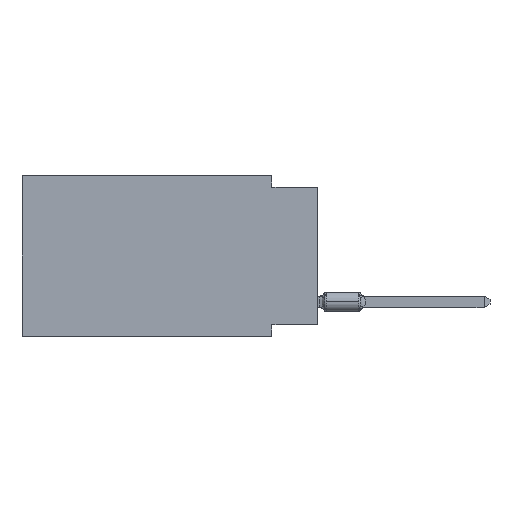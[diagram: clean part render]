
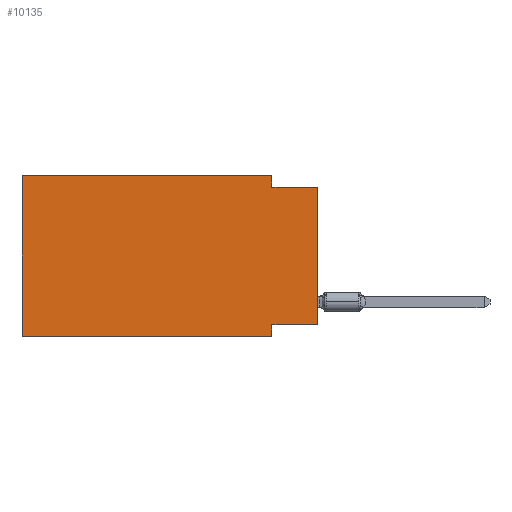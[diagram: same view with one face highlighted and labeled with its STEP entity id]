
A CAD part, left-side view. The second image highlights one B-rep face of the part: STEP entity #10135.
In plain terms, the highlighted planar face has unit normal (-1, 0, 0).
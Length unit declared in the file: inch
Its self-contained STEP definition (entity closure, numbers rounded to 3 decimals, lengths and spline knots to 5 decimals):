
#41 = DIRECTION ( 'NONE',  ( 0., -1., 0. ) ) ;
#230 = VERTEX_POINT ( 'NONE', #11716 ) ;
#420 = EDGE_CURVE ( 'NONE', #8386, #13280, #3571, .T. ) ;
#436 = VECTOR ( 'NONE', #15864, 39.37008 ) ;
#943 = VECTOR ( 'NONE', #9001, 39.37008 ) ;
#1126 = EDGE_CURVE ( 'NONE', #4996, #8189, #6018, .T. ) ;
#1551 = CARTESIAN_POINT ( 'NONE',  ( 0., 0.645, -0.35 ) ) ;
#1991 = DIRECTION ( 'NONE',  ( 1., 0., 0. ) ) ;
#2136 = LINE ( 'NONE', #11360, #19121 ) ;
#2369 = DIRECTION ( 'NONE',  ( 0., 1., 0. ) ) ;
#3134 = ORIENTED_EDGE ( 'NONE', *, *, #5900, .F. ) ;
#3478 = PLANE ( 'NONE',  #10831 ) ;
#3571 = LINE ( 'NONE', #9809, #436 ) ;
#3757 = LINE ( 'NONE', #15960, #12764 ) ;
#3804 = DIRECTION ( 'NONE',  ( 0., -1., 0. ) ) ;
#4207 = VECTOR ( 'NONE', #17292, 39.37008 ) ;
#4454 = CARTESIAN_POINT ( 'NONE',  ( 0., 0., -0.025 ) ) ;
#4685 = CARTESIAN_POINT ( 'NONE',  ( 0., 0.1, 0. ) ) ;
#4996 = VERTEX_POINT ( 'NONE', #9636 ) ;
#5167 = VECTOR ( 'NONE', #13246, 39.37008 ) ;
#5218 = VERTEX_POINT ( 'NONE', #12979 ) ;
#5900 = EDGE_CURVE ( 'NONE', #4996, #8386, #10203, .T. ) ;
#6018 = LINE ( 'NONE', #1551, #15182 ) ;
#7152 = VERTEX_POINT ( 'NONE', #4454 ) ;
#7201 = CARTESIAN_POINT ( 'NONE',  ( 0., 0., 0. ) ) ;
#7700 = ORIENTED_EDGE ( 'NONE', *, *, #17992, .F. ) ;
#7733 = CARTESIAN_POINT ( 'NONE',  ( 0., 0.1, -0.325 ) ) ;
#8189 = VERTEX_POINT ( 'NONE', #10014 ) ;
#8341 = CARTESIAN_POINT ( 'NONE',  ( 0., 0.1, -0.35 ) ) ;
#8386 = VERTEX_POINT ( 'NONE', #16266 ) ;
#8411 = ORIENTED_EDGE ( 'NONE', *, *, #1126, .T. ) ;
#8576 = LINE ( 'NONE', #7201, #5167 ) ;
#8704 = CARTESIAN_POINT ( 'NONE',  ( 0., 0.645, 0. ) ) ;
#9001 = DIRECTION ( 'NONE',  ( 0., 0., 1. ) ) ;
#9636 = CARTESIAN_POINT ( 'NONE',  ( 0., 0.645, -0.35 ) ) ;
#9748 = LINE ( 'NONE', #14316, #19417 ) ;
#9809 = CARTESIAN_POINT ( 'NONE',  ( 0., 0.645, 0. ) ) ;
#9934 = LINE ( 'NONE', #8341, #4207 ) ;
#9982 = DIRECTION ( 'NONE',  ( 0., 0., -1. ) ) ;
#10014 = CARTESIAN_POINT ( 'NONE',  ( 0., 0.1, -0.35 ) ) ;
#10135 = ADVANCED_FACE ( 'NONE', ( #11022 ), #3478, .F. ) ;
#10203 = LINE ( 'NONE', #8704, #943 ) ;
#10444 = VERTEX_POINT ( 'NONE', #7733 ) ;
#10776 = EDGE_LOOP ( 'NONE', ( #19668, #7700, #19240, #18719, #3134, #8411, #11526, #12096 ) ) ;
#10831 = AXIS2_PLACEMENT_3D ( 'NONE', #15583, #1991, #14689 ) ;
#11022 = FACE_OUTER_BOUND ( 'NONE', #10776, .T. ) ;
#11059 = EDGE_CURVE ( 'NONE', #13280, #5218, #2136, .T. ) ;
#11360 = CARTESIAN_POINT ( 'NONE',  ( 0., 0.1, 0. ) ) ;
#11526 = ORIENTED_EDGE ( 'NONE', *, *, #18346, .F. ) ;
#11716 = CARTESIAN_POINT ( 'NONE',  ( 0., 0., -0.325 ) ) ;
#11810 = EDGE_CURVE ( 'NONE', #230, #10444, #3757, .T. ) ;
#12096 = ORIENTED_EDGE ( 'NONE', *, *, #11810, .F. ) ;
#12764 = VECTOR ( 'NONE', #2369, 39.37008 ) ;
#12979 = CARTESIAN_POINT ( 'NONE',  ( 0., 0.1, -0.025 ) ) ;
#13246 = DIRECTION ( 'NONE',  ( 0., 0., 1. ) ) ;
#13280 = VERTEX_POINT ( 'NONE', #4685 ) ;
#14316 = CARTESIAN_POINT ( 'NONE',  ( 0., 0., -0.025 ) ) ;
#14689 = DIRECTION ( 'NONE',  ( 0., 0., -1. ) ) ;
#15182 = VECTOR ( 'NONE', #41, 39.37008 ) ;
#15583 = CARTESIAN_POINT ( 'NONE',  ( 0., 0.645, 0. ) ) ;
#15864 = DIRECTION ( 'NONE',  ( 0., -1., 0. ) ) ;
#15960 = CARTESIAN_POINT ( 'NONE',  ( 0., 0., -0.325 ) ) ;
#16266 = CARTESIAN_POINT ( 'NONE',  ( 0., 0.645, 0. ) ) ;
#16766 = EDGE_CURVE ( 'NONE', #230, #7152, #8576, .T. ) ;
#17292 = DIRECTION ( 'NONE',  ( 0., 0., -1. ) ) ;
#17992 = EDGE_CURVE ( 'NONE', #5218, #7152, #9748, .T. ) ;
#18346 = EDGE_CURVE ( 'NONE', #10444, #8189, #9934, .T. ) ;
#18719 = ORIENTED_EDGE ( 'NONE', *, *, #420, .F. ) ;
#19121 = VECTOR ( 'NONE', #9982, 39.37008 ) ;
#19240 = ORIENTED_EDGE ( 'NONE', *, *, #11059, .F. ) ;
#19417 = VECTOR ( 'NONE', #3804, 39.37008 ) ;
#19668 = ORIENTED_EDGE ( 'NONE', *, *, #16766, .T. ) ;
